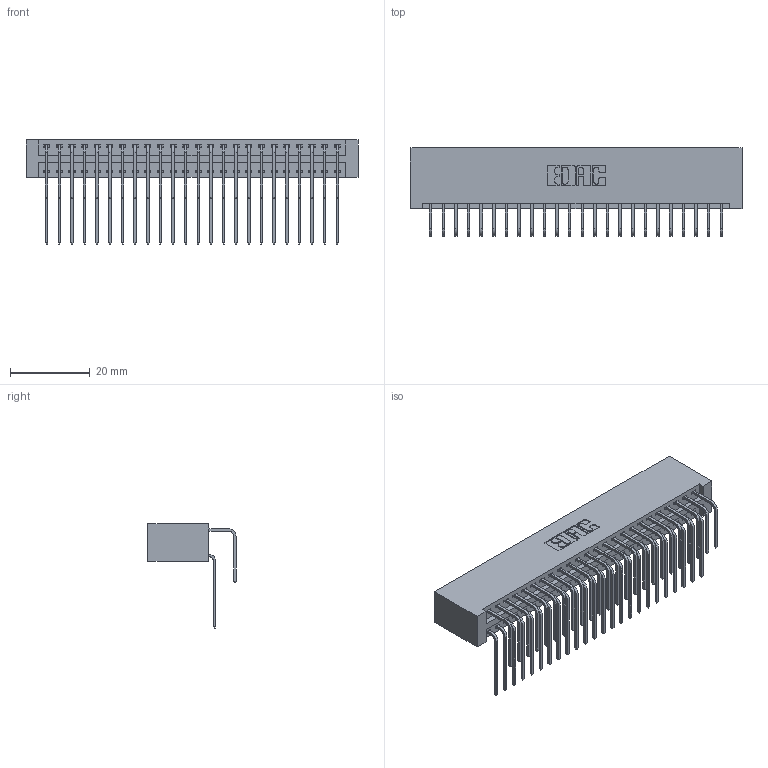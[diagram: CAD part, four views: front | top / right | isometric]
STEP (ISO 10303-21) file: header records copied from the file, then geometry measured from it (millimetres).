
FILE_DESCRIPTION (( 'STEP AP203' ), '1' );
FILE_NAME ('346-048-558-201.STEP', '2018-08-25T10:41:49', ( '' ), ( '' ), 'SwSTEP 2.0', 'SolidWorks 2016', '' );
FILE_SCHEMA (( 'CONFIG_CONTROL_DESIGN' ));
Length unit declared in the file: inch
Products named in the file (4): 346 Part_No Mounting Lugs; 345-292-001_558 559 Tail - 1; 345-292-001_558 Tail - 2; 346-048-558-201
Assembly tree (49 placements, depth 2):
  346-048-558-201
    346 Part_No Mounting Lugs
    345-292-001_558 559 Tail - 1  x24
    345-292-001_558 Tail - 2  x24
Bounding box: 83.44 x 22.16 x 26.16 mm (x, y, z)
Volume: 8846.7 mm3; surface area: 13369.1 mm2
Topology: 49 solids, 49 shells, 2706 faces, 8033 edges, 5290 vertices
Faces by surface type: plane 1848, cylinder 858
Entity records: 19593 total; most frequent: CARTESIAN_POINT 3303, ORIENTED_EDGE 3186, DIRECTION 2929, EDGE_CURVE 1593, LINE 1333, VECTOR 1333, VERTEX_POINT 1058, AXIS2_PLACEMENT_3D 798
